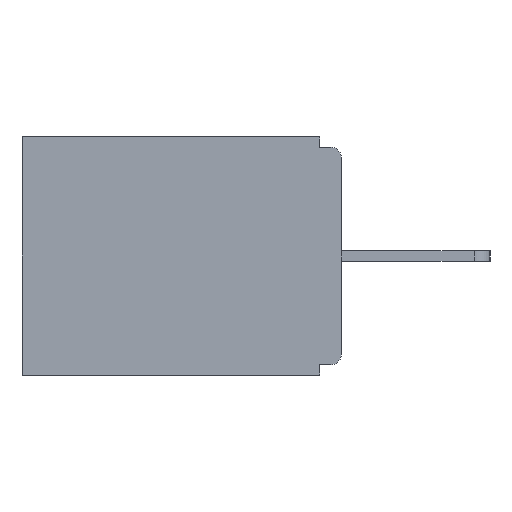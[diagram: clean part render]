
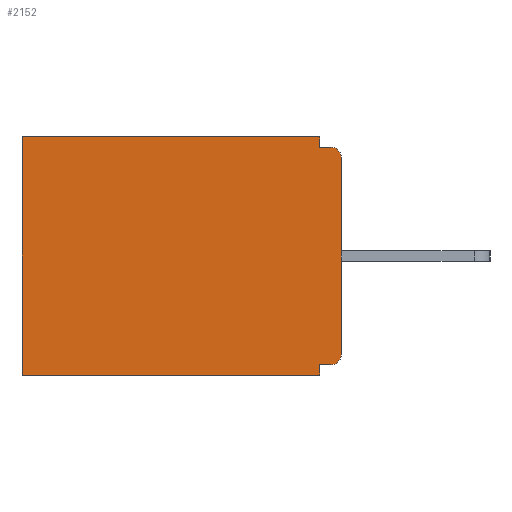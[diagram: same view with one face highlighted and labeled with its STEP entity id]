
A CAD part, left-side view. The second image highlights one B-rep face of the part: STEP entity #2152.
In plain terms, the highlighted planar face has unit normal (-1, 0, 0).
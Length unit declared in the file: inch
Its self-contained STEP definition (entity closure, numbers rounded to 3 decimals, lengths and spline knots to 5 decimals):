
#138 = ORIENTED_EDGE ( 'NONE', *, *, #10600, .F. ) ;
#259 = ORIENTED_EDGE ( 'NONE', *, *, #2631, .T. ) ;
#296 = ORIENTED_EDGE ( 'NONE', *, *, #9042, .T. ) ;
#652 = ORIENTED_EDGE ( 'NONE', *, *, #755, .F. ) ;
#755 = EDGE_CURVE ( 'NONE', #7829, #12092, #7070, .T. ) ;
#768 = VERTEX_POINT ( 'NONE', #6309 ) ;
#863 = VECTOR ( 'NONE', #3412, 39.37008 ) ;
#1378 = VECTOR ( 'NONE', #10760, 39.37008 ) ;
#1544 = LINE ( 'NONE', #6684, #9081 ) ;
#1737 = EDGE_CURVE ( 'NONE', #3942, #10116, #7491, .T. ) ;
#1735 = AXIS2_PLACEMENT_3D ( 'NONE', #1822, #1811, #2174 ) ;
#1811 = DIRECTION ( 'NONE',  ( -1., 0., 0. ) ) ;
#1822 = CARTESIAN_POINT ( 'NONE',  ( 0.298, 0.015, -0.313 ) ) ;
#1967 = EDGE_CURVE ( 'NONE', #7180, #6964, #11472, .T. ) ;
#2002 = ORIENTED_EDGE ( 'NONE', *, *, #9920, .T. ) ;
#2152 = ADVANCED_FACE ( 'NONE', ( #9364 ), #7436, .F. ) ;
#2174 = DIRECTION ( 'NONE',  ( 0., 0., -1. ) ) ;
#2327 = ORIENTED_EDGE ( 'NONE', *, *, #1737, .T. ) ;
#2390 = CARTESIAN_POINT ( 'NONE',  ( 0.298, 0.031, 0. ) ) ;
#2517 = LINE ( 'NONE', #6738, #4937 ) ;
#2528 = CARTESIAN_POINT ( 'NONE',  ( 0.298, 0., -0.313 ) ) ;
#2631 = EDGE_CURVE ( 'NONE', #7180, #768, #3696, .T. ) ;
#2877 = CARTESIAN_POINT ( 'NONE',  ( 0.298, 0.031, -0.343 ) ) ;
#2892 = DIRECTION ( 'NONE',  ( 0., 0., -1. ) ) ;
#3277 = CARTESIAN_POINT ( 'NONE',  ( 0.298, 0., 0. ) ) ;
#3384 = CARTESIAN_POINT ( 'NONE',  ( 0.298, 0.46, -0.343 ) ) ;
#3394 = DIRECTION ( 'NONE',  ( 0., 1., 0. ) ) ;
#3412 = DIRECTION ( 'NONE',  ( 0., 1., 0. ) ) ;
#3629 = DIRECTION ( 'NONE',  ( 0., 0., -1. ) ) ;
#3696 = LINE ( 'NONE', #3277, #863 ) ;
#3710 = DIRECTION ( 'NONE',  ( 0., -1., 0. ) ) ;
#3942 = VERTEX_POINT ( 'NONE', #7522 ) ;
#4010 = EDGE_CURVE ( 'NONE', #6964, #10116, #2517, .T. ) ;
#4185 = LINE ( 'NONE', #8849, #8946 ) ;
#4861 = LINE ( 'NONE', #11834, #9546 ) ;
#4937 = VECTOR ( 'NONE', #3710, 39.37008 ) ;
#5041 = VERTEX_POINT ( 'NONE', #2528 ) ;
#5147 = AXIS2_PLACEMENT_3D ( 'NONE', #7340, #9663, #3629 ) ;
#5148 = DIRECTION ( 'NONE',  ( 0., 1., 0. ) ) ;
#5364 = ORIENTED_EDGE ( 'NONE', *, *, #9969, .F. ) ;
#5436 = LINE ( 'NONE', #7816, #7635 ) ;
#6099 = CARTESIAN_POINT ( 'NONE',  ( 0.298, 0.015, -0.328 ) ) ;
#6309 = CARTESIAN_POINT ( 'NONE',  ( 0.298, 0.46, 0. ) ) ;
#6311 = CARTESIAN_POINT ( 'NONE',  ( 0.298, 0.031, -0.328 ) ) ;
#6422 = CARTESIAN_POINT ( 'NONE',  ( 0.298, 0.031, -0.343 ) ) ;
#6684 = CARTESIAN_POINT ( 'NONE',  ( 0.298, 0., -0.328 ) ) ;
#6738 = CARTESIAN_POINT ( 'NONE',  ( 0.298, 0., -0.015 ) ) ;
#6939 = ORIENTED_EDGE ( 'NONE', *, *, #9865, .F. ) ;
#6964 = VERTEX_POINT ( 'NONE', #8302 ) ;
#6965 = ORIENTED_EDGE ( 'NONE', *, *, #1967, .F. ) ;
#7051 = CARTESIAN_POINT ( 'NONE',  ( 0.298, 0.031, -0.343 ) ) ;
#7070 = LINE ( 'NONE', #2877, #11503 ) ;
#7180 = VERTEX_POINT ( 'NONE', #2390 ) ;
#7330 = ORIENTED_EDGE ( 'NONE', *, *, #4010, .F. ) ;
#7340 = CARTESIAN_POINT ( 'NONE',  ( 0.298, 0., 0. ) ) ;
#7436 = PLANE ( 'NONE',  #5147 ) ;
#7491 = CIRCLE ( 'NONE', #7508, 0.015 ) ;
#7508 = AXIS2_PLACEMENT_3D ( 'NONE', #10541, #10706, #9217 ) ;
#7522 = CARTESIAN_POINT ( 'NONE',  ( 0.298, 0., -0.03 ) ) ;
#7635 = VECTOR ( 'NONE', #5148, 39.37008 ) ;
#7816 = CARTESIAN_POINT ( 'NONE',  ( 0.298, 0., -0.343 ) ) ;
#7829 = VERTEX_POINT ( 'NONE', #6311 ) ;
#8302 = CARTESIAN_POINT ( 'NONE',  ( 0.298, 0.031, -0.015 ) ) ;
#8849 = CARTESIAN_POINT ( 'NONE',  ( 0.298, 0., 0. ) ) ;
#8946 = VECTOR ( 'NONE', #9064, 39.37008 ) ;
#9042 = EDGE_CURVE ( 'NONE', #768, #9142, #4861, .T. ) ;
#9064 = DIRECTION ( 'NONE',  ( 0., 0., -1. ) ) ;
#9081 = VECTOR ( 'NONE', #3394, 39.37008 ) ;
#9142 = VERTEX_POINT ( 'NONE', #3384 ) ;
#9217 = DIRECTION ( 'NONE',  ( 0., 0., -1. ) ) ;
#9364 = FACE_OUTER_BOUND ( 'NONE', #12177, .T. ) ;
#9546 = VECTOR ( 'NONE', #11642, 39.37008 ) ;
#9663 = DIRECTION ( 'NONE',  ( 1., 0., 0. ) ) ;
#9865 = EDGE_CURVE ( 'NONE', #12092, #9142, #5436, .T. ) ;
#9920 = EDGE_CURVE ( 'NONE', #11872, #5041, #11763, .T. ) ;
#9969 = EDGE_CURVE ( 'NONE', #3942, #5041, #4185, .T. ) ;
#10116 = VERTEX_POINT ( 'NONE', #11057 ) ;
#10541 = CARTESIAN_POINT ( 'NONE',  ( 0.298, 0.015, -0.03 ) ) ;
#10600 = EDGE_CURVE ( 'NONE', #11872, #7829, #1544, .T. ) ;
#10706 = DIRECTION ( 'NONE',  ( -1., 0., 0. ) ) ;
#10760 = DIRECTION ( 'NONE',  ( 0., 0., -1. ) ) ;
#11057 = CARTESIAN_POINT ( 'NONE',  ( 0.298, 0.015, -0.015 ) ) ;
#11472 = LINE ( 'NONE', #7051, #1378 ) ;
#11503 = VECTOR ( 'NONE', #2892, 39.37008 ) ;
#11642 = DIRECTION ( 'NONE',  ( 0., 0., -1. ) ) ;
#11763 = CIRCLE ( 'NONE', #1735, 0.015 ) ;
#11834 = CARTESIAN_POINT ( 'NONE',  ( 0.298, 0.46, 0. ) ) ;
#11872 = VERTEX_POINT ( 'NONE', #6099 ) ;
#12092 = VERTEX_POINT ( 'NONE', #6422 ) ;
#12177 = EDGE_LOOP ( 'NONE', ( #2327, #7330, #6965, #259, #296, #6939, #652, #138, #2002, #5364 ) ) ;
